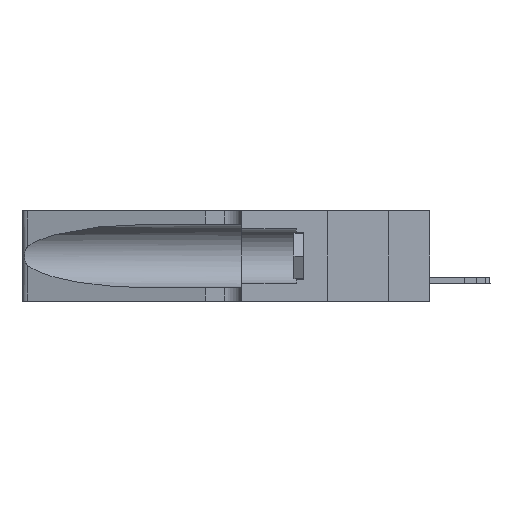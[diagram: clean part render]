
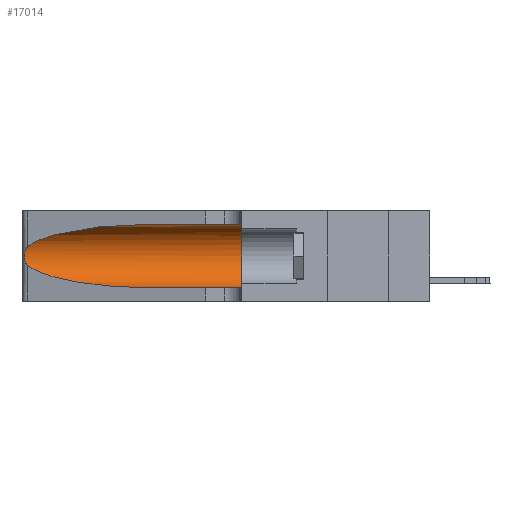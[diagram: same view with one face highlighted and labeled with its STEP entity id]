
A CAD part, left-side view. The second image highlights one B-rep face of the part: STEP entity #17014.
In plain terms, the highlighted cylindrical face has radius 3.308 mm (diameter 6.617 mm), a partial arc.
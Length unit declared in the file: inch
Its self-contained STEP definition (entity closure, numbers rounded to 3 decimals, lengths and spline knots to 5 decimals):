
#180 = CARTESIAN_POINT ( 'NONE',  ( 0.25787, 1.23484, 0.2124 ) ) ;
#190 = CARTESIAN_POINT ( 'NONE',  ( 0.1305, 0.35, 0.05475 ) ) ;
#264 = CARTESIAN_POINT ( 'NONE',  ( 0.25854, 1.2359, 0.20912 ) ) ;
#344 = CARTESIAN_POINT ( 'NONE',  ( 0.18966, 0.96281, 0.05475 ) ) ;
#433 = CARTESIAN_POINT ( 'NONE',  ( 0.25639, 1.23186, 0.15144 ) ) ;
#1318 = EDGE_CURVE ( 'NONE', #10736, #8700, #18585, .T. ) ;
#1456 = AXIS2_PLACEMENT_3D ( 'NONE', #1583, #9162, #22446 ) ;
#1583 = CARTESIAN_POINT ( 'NONE',  ( 0.1305, 0.35, 0.185 ) ) ;
#2610 = EDGE_LOOP ( 'NONE', ( #9525, #16287, #22559, #23419, #5280, #18326 ) ) ;
#3977 = CARTESIAN_POINT ( 'NONE',  ( 0.25856, 1.23593, 0.16098 ) ) ;
#4127 = CARTESIAN_POINT ( 'NONE',  ( 0.25487, 1.22718, 0.14631 ) ) ;
#4311 =( BOUNDED_CURVE ( )  B_SPLINE_CURVE ( 3, ( #4127, #8085, #344, #5935 ),
 .UNSPECIFIED., .F., .F. ) 
 B_SPLINE_CURVE_WITH_KNOTS ( ( 4, 4 ),
 ( 3.44316, 4.71239 ),
 .UNSPECIFIED. ) 
 CURVE ( )  GEOMETRIC_REPRESENTATION_ITEM ( )  RATIONAL_B_SPLINE_CURVE ( ( 1., 0.87, 0.87, 1. ) ) 
 REPRESENTATION_ITEM ( '' )  );
#4861 = EDGE_CURVE ( 'NONE', #21968, #14031, #4311, .T. ) ;
#4994 = CARTESIAN_POINT ( 'NONE',  ( 0.1305, 0.72297, 0.05475 ) ) ;
#5280 = ORIENTED_EDGE ( 'NONE', *, *, #12023, .F. ) ;
#5506 =( BOUNDED_CURVE ( )  B_SPLINE_CURVE ( 3, ( #16186, #16103, #15853, #12054 ),
 .UNSPECIFIED., .F., .T. ) 
 B_SPLINE_CURVE_WITH_KNOTS ( ( 4, 4 ),
 ( 1.5708, 2.84003 ),
 .UNSPECIFIED. ) 
 CURVE ( )  GEOMETRIC_REPRESENTATION_ITEM ( )  RATIONAL_B_SPLINE_CURVE ( ( 1., 0.87, 0.87, 1. ) ) 
 REPRESENTATION_ITEM ( '' )  );
#5935 = CARTESIAN_POINT ( 'NONE',  ( 0.1305, 0.72297, 0.05475 ) ) ;
#6270 = B_SPLINE_CURVE_WITH_KNOTS ( 'NONE', 3,
 ( #11510, #21132, #13600, #180, #264, #9603, #7921, #9516, #13521, #3977, #9759, #433, #19321, #7764 ),
 .UNSPECIFIED., .F., .F.,
 ( 4, 2, 2, 2, 2, 2, 4 ),
 ( 0., 0.00027, 0.00053, 0.00107, 0.0016, 0.00187, 0.00214 ),
 .UNSPECIFIED. ) ;
#6417 = CYLINDRICAL_SURFACE ( 'NONE', #22166, 0.13025 ) ;
#7222 = CIRCLE ( 'NONE', #1456, 0.13025 ) ;
#7227 = CARTESIAN_POINT ( 'NONE',  ( 0.1305, 0.72297, 0.31525 ) ) ;
#7764 = CARTESIAN_POINT ( 'NONE',  ( 0.25487, 1.22718, 0.14631 ) ) ;
#7921 = CARTESIAN_POINT ( 'NONE',  ( 0.26075, 1.23896, 0.19203 ) ) ;
#8085 = CARTESIAN_POINT ( 'NONE',  ( 0.2373, 1.15595, 0.08982 ) ) ;
#8329 = VERTEX_POINT ( 'NONE', #10798 ) ;
#8357 = DIRECTION ( 'NONE',  ( 0., -1., 0. ) ) ;
#8700 = VERTEX_POINT ( 'NONE', #13351 ) ;
#9162 = DIRECTION ( 'NONE',  ( 0., 1., 0. ) ) ;
#9516 = CARTESIAN_POINT ( 'NONE',  ( 0.26075, 1.23896, 0.178 ) ) ;
#9525 = ORIENTED_EDGE ( 'NONE', *, *, #18385, .T. ) ;
#9603 = CARTESIAN_POINT ( 'NONE',  ( 0.26018, 1.23835, 0.19895 ) ) ;
#9759 = CARTESIAN_POINT ( 'NONE',  ( 0.25789, 1.23486, 0.15765 ) ) ;
#9949 = DIRECTION ( 'NONE',  ( 0., 0., -1. ) ) ;
#10736 = VERTEX_POINT ( 'NONE', #7227 ) ;
#10798 = CARTESIAN_POINT ( 'NONE',  ( 0.25487, 1.22718, 0.22369 ) ) ;
#11510 = CARTESIAN_POINT ( 'NONE',  ( 0.25487, 1.22718, 0.22369 ) ) ;
#11597 = LINE ( 'NONE', #14785, #19916 ) ;
#12023 = EDGE_CURVE ( 'NONE', #8700, #22918, #7222, .T. ) ;
#12054 = CARTESIAN_POINT ( 'NONE',  ( 0.25487, 1.22718, 0.22369 ) ) ;
#12964 = FACE_OUTER_BOUND ( 'NONE', #2610, .T. ) ;
#13351 = CARTESIAN_POINT ( 'NONE',  ( 0.1305, 0.35, 0.31525 ) ) ;
#13521 = CARTESIAN_POINT ( 'NONE',  ( 0.26017, 1.23833, 0.17102 ) ) ;
#13600 = CARTESIAN_POINT ( 'NONE',  ( 0.25639, 1.23184, 0.21858 ) ) ;
#14031 = VERTEX_POINT ( 'NONE', #4994 ) ;
#14785 = CARTESIAN_POINT ( 'NONE',  ( 0.1305, 1.61858, 0.05475 ) ) ;
#14960 = VECTOR ( 'NONE', #21941, 39.37008 ) ;
#14975 = EDGE_CURVE ( 'NONE', #8329, #21968, #6270, .T. ) ;
#15853 = CARTESIAN_POINT ( 'NONE',  ( 0.2373, 1.15595, 0.28018 ) ) ;
#15916 = CARTESIAN_POINT ( 'NONE',  ( 0.1305, 1.61858, 0.185 ) ) ;
#16103 = CARTESIAN_POINT ( 'NONE',  ( 0.18966, 0.96281, 0.31525 ) ) ;
#16186 = CARTESIAN_POINT ( 'NONE',  ( 0.1305, 0.72297, 0.31525 ) ) ;
#16287 = ORIENTED_EDGE ( 'NONE', *, *, #14975, .T. ) ;
#16307 = CARTESIAN_POINT ( 'NONE',  ( 0.1305, 1.61858, 0.31525 ) ) ;
#17014 = ADVANCED_FACE ( 'NONE', ( #12964 ), #6417, .F. ) ;
#17062 = DIRECTION ( 'NONE',  ( 0., -1., 0. ) ) ;
#18326 = ORIENTED_EDGE ( 'NONE', *, *, #1318, .F. ) ;
#18385 = EDGE_CURVE ( 'NONE', #10736, #8329, #5506, .T. ) ;
#18585 = LINE ( 'NONE', #16307, #14960 ) ;
#19321 = CARTESIAN_POINT ( 'NONE',  ( 0.25555, 1.22993, 0.14849 ) ) ;
#19916 = VECTOR ( 'NONE', #17062, 39.37008 ) ;
#20202 = CARTESIAN_POINT ( 'NONE',  ( 0.25487, 1.22718, 0.14631 ) ) ;
#21132 = CARTESIAN_POINT ( 'NONE',  ( 0.25555, 1.22994, 0.2215 ) ) ;
#21143 = EDGE_CURVE ( 'NONE', #14031, #22918, #11597, .T. ) ;
#21941 = DIRECTION ( 'NONE',  ( 0., -1., 0. ) ) ;
#21968 = VERTEX_POINT ( 'NONE', #20202 ) ;
#22166 = AXIS2_PLACEMENT_3D ( 'NONE', #15916, #8357, #9949 ) ;
#22446 = DIRECTION ( 'NONE',  ( 0., 0., 1. ) ) ;
#22559 = ORIENTED_EDGE ( 'NONE', *, *, #4861, .T. ) ;
#22918 = VERTEX_POINT ( 'NONE', #190 ) ;
#23419 = ORIENTED_EDGE ( 'NONE', *, *, #21143, .T. ) ;
